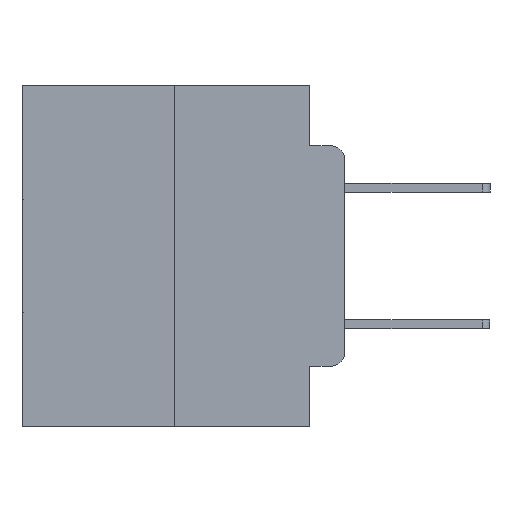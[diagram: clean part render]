
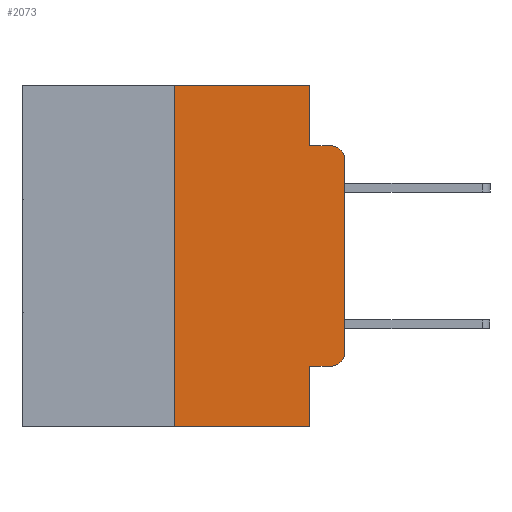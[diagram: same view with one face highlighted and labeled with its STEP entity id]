
A CAD part, left-side view. The second image highlights one B-rep face of the part: STEP entity #2073.
In plain terms, the highlighted planar face has unit normal (-1, 0, 0).
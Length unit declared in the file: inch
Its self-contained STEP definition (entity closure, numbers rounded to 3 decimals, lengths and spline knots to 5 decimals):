
#23 = EDGE_CURVE ( 'NONE', #22350, #24813, #3701, .T. ) ;
#868 = DIRECTION ( 'NONE',  ( 0., 0., -1. ) ) ;
#1610 = VERTEX_POINT ( 'NONE', #17698 ) ;
#1851 = ORIENTED_EDGE ( 'NONE', *, *, #8146, .F. ) ;
#2073 = ADVANCED_FACE ( 'NONE', ( #7206 ), #15231, .F. ) ;
#2426 = EDGE_CURVE ( 'NONE', #1610, #14695, #25238, .T. ) ;
#2954 = LINE ( 'NONE', #7450, #24678 ) ;
#2970 = DIRECTION ( 'NONE',  ( 0., -1., 0. ) ) ;
#3084 = AXIS2_PLACEMENT_3D ( 'NONE', #26154, #13671, #868 ) ;
#3500 = CARTESIAN_POINT ( 'NONE',  ( 0., 0.051, 0. ) ) ;
#3503 = CARTESIAN_POINT ( 'NONE',  ( 0., 0.051, -0.0885 ) ) ;
#3701 = LINE ( 'NONE', #5714, #14287 ) ;
#3856 = DIRECTION ( 'NONE',  ( 0., 0., 1. ) ) ;
#4181 = LINE ( 'NONE', #7532, #9126 ) ;
#5333 = EDGE_CURVE ( 'NONE', #1610, #10857, #6728, .T. ) ;
#5714 = CARTESIAN_POINT ( 'NONE',  ( 0., 0.473, 0. ) ) ;
#6106 = VECTOR ( 'NONE', #13495, 39.37008 ) ;
#6728 = LINE ( 'NONE', #19736, #6106 ) ;
#7013 = ORIENTED_EDGE ( 'NONE', *, *, #2426, .T. ) ;
#7206 = FACE_OUTER_BOUND ( 'NONE', #16779, .T. ) ;
#7340 = VERTEX_POINT ( 'NONE', #13875 ) ;
#7450 = CARTESIAN_POINT ( 'NONE',  ( 0., 0.473, -0.5 ) ) ;
#7532 = CARTESIAN_POINT ( 'NONE',  ( 0., 0., 0. ) ) ;
#7745 = CARTESIAN_POINT ( 'NONE',  ( 0., 0.473, 0. ) ) ;
#7985 = EDGE_CURVE ( 'NONE', #21300, #10857, #2954, .T. ) ;
#8146 = EDGE_CURVE ( 'NONE', #21300, #22350, #15225, .T. ) ;
#8484 = CIRCLE ( 'NONE', #16468, 0.02 ) ;
#8645 = CARTESIAN_POINT ( 'NONE',  ( 0., 0.02, -0.4115 ) ) ;
#8837 = VERTEX_POINT ( 'NONE', #16677 ) ;
#9126 = VECTOR ( 'NONE', #20239, 39.37008 ) ;
#9183 = DIRECTION ( 'NONE',  ( -1., 0., 0. ) ) ;
#9409 = ORIENTED_EDGE ( 'NONE', *, *, #15245, .T. ) ;
#9516 = ORIENTED_EDGE ( 'NONE', *, *, #23, .F. ) ;
#9540 = CARTESIAN_POINT ( 'NONE',  ( 0., 0.25, -0.5 ) ) ;
#10582 = LINE ( 'NONE', #3503, #21083 ) ;
#10857 = VERTEX_POINT ( 'NONE', #18320 ) ;
#11461 = DIRECTION ( 'NONE',  ( 0., 0., -1. ) ) ;
#12410 = EDGE_CURVE ( 'NONE', #24813, #25291, #13590, .T. ) ;
#12620 = ORIENTED_EDGE ( 'NONE', *, *, #12410, .F. ) ;
#13184 = ORIENTED_EDGE ( 'NONE', *, *, #5333, .F. ) ;
#13495 = DIRECTION ( 'NONE',  ( 0., 0., -1. ) ) ;
#13590 = LINE ( 'NONE', #23994, #18529 ) ;
#13671 = DIRECTION ( 'NONE',  ( -1., 0., 0. ) ) ;
#13813 = EDGE_CURVE ( 'NONE', #25291, #24886, #10582, .T. ) ;
#13875 = CARTESIAN_POINT ( 'NONE',  ( 0., 0., -0.1085 ) ) ;
#14152 = VECTOR ( 'NONE', #17396, 39.37008 ) ;
#14287 = VECTOR ( 'NONE', #2970, 39.37008 ) ;
#14391 = CARTESIAN_POINT ( 'NONE',  ( 0., 0.25, 0. ) ) ;
#14394 = DIRECTION ( 'NONE',  ( 1., 0., 0. ) ) ;
#14695 = VERTEX_POINT ( 'NONE', #8645 ) ;
#14762 = CARTESIAN_POINT ( 'NONE',  ( 0., 0.051, -0.4115 ) ) ;
#14787 = ORIENTED_EDGE ( 'NONE', *, *, #13813, .F. ) ;
#15225 = LINE ( 'NONE', #14391, #20132 ) ;
#15231 = PLANE ( 'NONE',  #17967 ) ;
#15245 = EDGE_CURVE ( 'NONE', #7340, #24886, #8484, .T. ) ;
#15693 = ORIENTED_EDGE ( 'NONE', *, *, #25500, .T. ) ;
#16468 = AXIS2_PLACEMENT_3D ( 'NONE', #21771, #9183, #23858 ) ;
#16677 = CARTESIAN_POINT ( 'NONE',  ( 0., 0., -0.3915 ) ) ;
#16753 = DIRECTION ( 'NONE',  ( 0., 0., -1. ) ) ;
#16779 = EDGE_LOOP ( 'NONE', ( #22235, #9409, #14787, #12620, #9516, #1851, #21835, #13184, #7013, #15693 ) ) ;
#17396 = DIRECTION ( 'NONE',  ( 0., -1., 0. ) ) ;
#17698 = CARTESIAN_POINT ( 'NONE',  ( 0., 0.051, -0.4115 ) ) ;
#17967 = AXIS2_PLACEMENT_3D ( 'NONE', #7745, #14394, #16753 ) ;
#18320 = CARTESIAN_POINT ( 'NONE',  ( 0., 0.051, -0.5 ) ) ;
#18529 = VECTOR ( 'NONE', #11461, 39.37008 ) ;
#19457 = EDGE_CURVE ( 'NONE', #8837, #7340, #4181, .T. ) ;
#19736 = CARTESIAN_POINT ( 'NONE',  ( 0., 0.051, 0. ) ) ;
#20132 = VECTOR ( 'NONE', #3856, 39.37008 ) ;
#20239 = DIRECTION ( 'NONE',  ( 0., 0., 1. ) ) ;
#20380 = DIRECTION ( 'NONE',  ( 0., -1., 0. ) ) ;
#20648 = CARTESIAN_POINT ( 'NONE',  ( 0., 0.02, -0.0885 ) ) ;
#21083 = VECTOR ( 'NONE', #20380, 39.37008 ) ;
#21300 = VERTEX_POINT ( 'NONE', #9540 ) ;
#21600 = CARTESIAN_POINT ( 'NONE',  ( 0., 0.25, 0. ) ) ;
#21771 = CARTESIAN_POINT ( 'NONE',  ( 0., 0.02, -0.1085 ) ) ;
#21835 = ORIENTED_EDGE ( 'NONE', *, *, #7985, .T. ) ;
#22080 = CARTESIAN_POINT ( 'NONE',  ( 0., 0.051, -0.0885 ) ) ;
#22235 = ORIENTED_EDGE ( 'NONE', *, *, #19457, .T. ) ;
#22350 = VERTEX_POINT ( 'NONE', #21600 ) ;
#23858 = DIRECTION ( 'NONE',  ( 0., 0., -1. ) ) ;
#23994 = CARTESIAN_POINT ( 'NONE',  ( 0., 0.051, 0. ) ) ;
#24260 = DIRECTION ( 'NONE',  ( 0., -1., 0. ) ) ;
#24678 = VECTOR ( 'NONE', #24260, 39.37008 ) ;
#24813 = VERTEX_POINT ( 'NONE', #3500 ) ;
#24886 = VERTEX_POINT ( 'NONE', #20648 ) ;
#25238 = LINE ( 'NONE', #14762, #14152 ) ;
#25291 = VERTEX_POINT ( 'NONE', #22080 ) ;
#25500 = EDGE_CURVE ( 'NONE', #14695, #8837, #26239, .T. ) ;
#26154 = CARTESIAN_POINT ( 'NONE',  ( 0., 0.02, -0.3915 ) ) ;
#26239 = CIRCLE ( 'NONE', #3084, 0.02 ) ;
